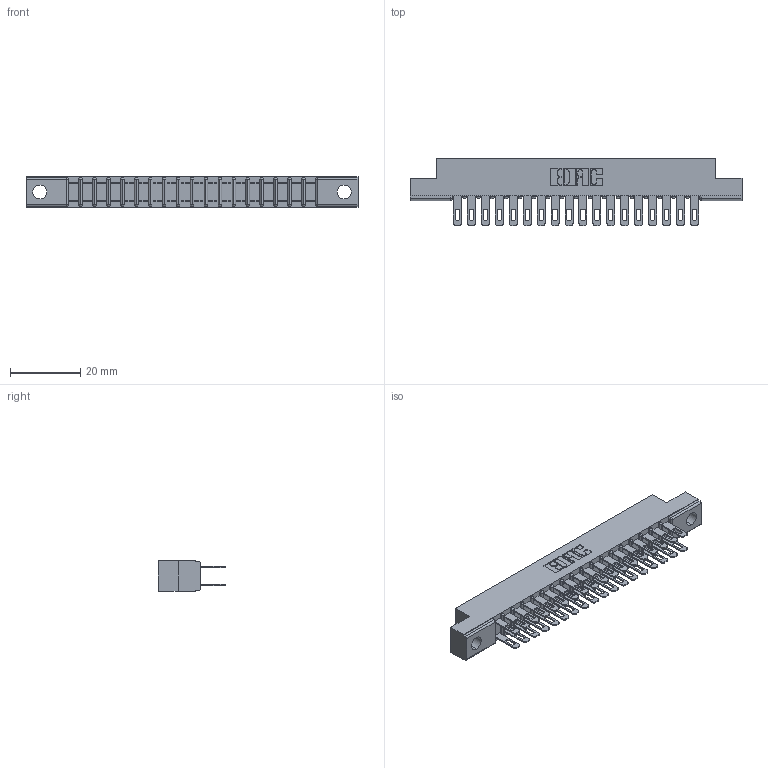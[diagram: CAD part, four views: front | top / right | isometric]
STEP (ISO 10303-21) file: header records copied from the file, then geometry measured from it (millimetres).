
FILE_DESCRIPTION (( 'STEP AP203' ), '1' );
FILE_NAME ('357-036-500-202.STEP', '2019-09-18T02:56:28', ( '' ), ( '' ), 'SwSTEP 2.0', 'SolidWorks 2016', '' );
FILE_SCHEMA (( 'CONFIG_CONTROL_DESIGN' ));
Length unit declared in the file: inch
Products named in the file (3): 307-290-001_500; 307 Part_.128 Dia Mounting Holes; 357-036-500-202
Assembly tree (37 placements, depth 2):
  357-036-500-202
    307 Part_.128 Dia Mounting Holes
    307-290-001_500  x36
Bounding box: 94.34 x 19.18 x 8.71 mm (x, y, z)
Volume: 6186.3 mm3; surface area: 11137 mm2
Topology: 37 solids, 37 shells, 1793 faces, 5003 edges, 3234 vertices
Faces by surface type: plane 1150, cylinder 605, sphere 38
Entity records: 18942 total; most frequent: CARTESIAN_POINT 3102, ORIENTED_EDGE 3070, DIRECTION 3051, EDGE_CURVE 1535, VECTOR 1165, LINE 1165, VERTEX_POINT 994, AXIS2_PLACEMENT_3D 943
